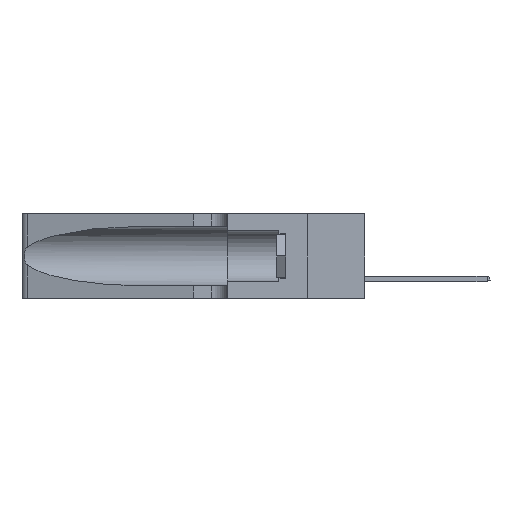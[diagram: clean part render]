
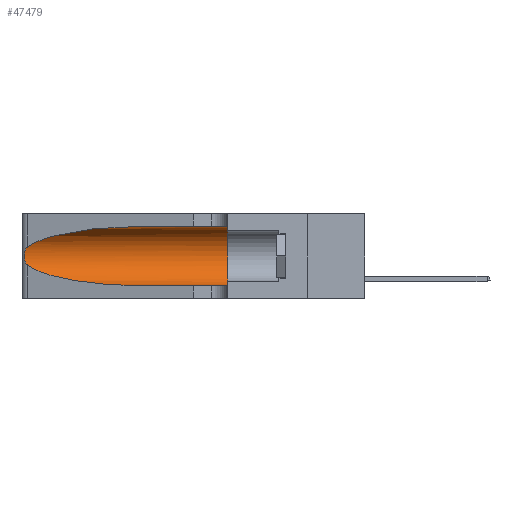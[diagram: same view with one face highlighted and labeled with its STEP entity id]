
A CAD part, left-side view. The second image highlights one B-rep face of the part: STEP entity #47479.
In plain terms, the highlighted cylindrical face has radius 3.308 mm (diameter 6.617 mm), a partial arc.
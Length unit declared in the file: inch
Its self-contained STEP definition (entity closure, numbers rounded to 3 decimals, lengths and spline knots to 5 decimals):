
#219 =( BOUNDED_CURVE ( )  B_SPLINE_CURVE ( 3, ( #15492, #26360, #33299, #37040 ),
 .UNSPECIFIED., .F., .T. ) 
 B_SPLINE_CURVE_WITH_KNOTS ( ( 4, 4 ),
 ( 1.5708, 2.84003 ),
 .UNSPECIFIED. ) 
 CURVE ( )  GEOMETRIC_REPRESENTATION_ITEM ( )  RATIONAL_B_SPLINE_CURVE ( ( 1., 0.87, 0.87, 1. ) ) 
 REPRESENTATION_ITEM ( '' )  );
#1433 = CARTESIAN_POINT ( 'NONE',  ( 0.2373, 1.15595, 0.08982 ) ) ;
#1579 = VERTEX_POINT ( 'NONE', #8436 ) ;
#2025 = DIRECTION ( 'NONE',  ( 0., 1., 0. ) ) ;
#2795 = ORIENTED_EDGE ( 'NONE', *, *, #7237, .F. ) ;
#5090 = LINE ( 'NONE', #26822, #35211 ) ;
#5856 = EDGE_CURVE ( 'NONE', #35575, #1579, #219, .T. ) ;
#6345 = CARTESIAN_POINT ( 'NONE',  ( 0.1305, 1.61858, 0.05475 ) ) ;
#6360 = FACE_OUTER_BOUND ( 'NONE', #33019, .T. ) ;
#6523 = ORIENTED_EDGE ( 'NONE', *, *, #47798, .F. ) ;
#6576 = CARTESIAN_POINT ( 'NONE',  ( 0.26017, 1.23833, 0.17102 ) ) ;
#6625 = DIRECTION ( 'NONE',  ( 0., -1., 0. ) ) ;
#6872 = CARTESIAN_POINT ( 'NONE',  ( 0.25555, 1.22993, 0.14849 ) ) ;
#7237 = EDGE_CURVE ( 'NONE', #11535, #20867, #25740, .T. ) ;
#8436 = CARTESIAN_POINT ( 'NONE',  ( 0.25487, 1.22718, 0.22369 ) ) ;
#9831 = EDGE_CURVE ( 'NONE', #43937, #15909, #36187, .T. ) ;
#10055 = AXIS2_PLACEMENT_3D ( 'NONE', #39849, #6625, #10306 ) ;
#10306 = DIRECTION ( 'NONE',  ( 0., 0., -1. ) ) ;
#10555 = CARTESIAN_POINT ( 'NONE',  ( 0.25789, 1.23486, 0.15765 ) ) ;
#11535 = VERTEX_POINT ( 'NONE', #21800 ) ;
#13190 = CARTESIAN_POINT ( 'NONE',  ( 0.25555, 1.22994, 0.2215 ) ) ;
#13523 = ORIENTED_EDGE ( 'NONE', *, *, #31975, .T. ) ;
#15492 = CARTESIAN_POINT ( 'NONE',  ( 0.1305, 0.72297, 0.31525 ) ) ;
#15909 = VERTEX_POINT ( 'NONE', #30723 ) ;
#16285 = CARTESIAN_POINT ( 'NONE',  ( 0.1305, 0.72297, 0.05475 ) ) ;
#16612 = CARTESIAN_POINT ( 'NONE',  ( 0.18966, 0.96281, 0.05475 ) ) ;
#16851 = DIRECTION ( 'NONE',  ( 0., 0., 1. ) ) ;
#18009 = CARTESIAN_POINT ( 'NONE',  ( 0.26018, 1.23835, 0.19895 ) ) ;
#18024 = ORIENTED_EDGE ( 'NONE', *, *, #45085, .T. ) ;
#19514 = CARTESIAN_POINT ( 'NONE',  ( 0.1305, 0.35, 0.05475 ) ) ;
#20793 = CYLINDRICAL_SURFACE ( 'NONE', #10055, 0.13025 ) ;
#20867 = VERTEX_POINT ( 'NONE', #19514 ) ;
#21800 = CARTESIAN_POINT ( 'NONE',  ( 0.1305, 0.35, 0.31525 ) ) ;
#22569 = ORIENTED_EDGE ( 'NONE', *, *, #5856, .T. ) ;
#24175 = CARTESIAN_POINT ( 'NONE',  ( 0.1305, 0.35, 0.185 ) ) ;
#24402 = CARTESIAN_POINT ( 'NONE',  ( 0.25854, 1.2359, 0.20912 ) ) ;
#25740 = CIRCLE ( 'NONE', #35718, 0.13025 ) ;
#25904 = CARTESIAN_POINT ( 'NONE',  ( 0.1305, 0.72297, 0.31525 ) ) ;
#26360 = CARTESIAN_POINT ( 'NONE',  ( 0.18966, 0.96281, 0.31525 ) ) ;
#26822 = CARTESIAN_POINT ( 'NONE',  ( 0.1305, 1.61858, 0.31525 ) ) ;
#27967 = CARTESIAN_POINT ( 'NONE',  ( 0.25487, 1.22718, 0.22369 ) ) ;
#28757 = CARTESIAN_POINT ( 'NONE',  ( 0.25487, 1.22718, 0.14631 ) ) ;
#28917 = CARTESIAN_POINT ( 'NONE',  ( 0.26075, 1.23896, 0.178 ) ) ;
#29241 = LINE ( 'NONE', #6345, #47222 ) ;
#30723 = CARTESIAN_POINT ( 'NONE',  ( 0.1305, 0.72297, 0.05475 ) ) ;
#31192 = CARTESIAN_POINT ( 'NONE',  ( 0.25487, 1.22718, 0.14631 ) ) ;
#31975 = EDGE_CURVE ( 'NONE', #15909, #20867, #29241, .T. ) ;
#32368 = B_SPLINE_CURVE_WITH_KNOTS ( 'NONE', 3,
 ( #27967, #13190, #43019, #46580, #24402, #18009, #47671, #28917, #6576, #40093, #10555, #47215, #6872, #28757 ),
 .UNSPECIFIED., .F., .F.,
 ( 4, 2, 2, 2, 2, 2, 4 ),
 ( 0., 0.00027, 0.00053, 0.00107, 0.0016, 0.00187, 0.00214 ),
 .UNSPECIFIED. ) ;
#32394 = DIRECTION ( 'NONE',  ( 0., -1., 0. ) ) ;
#33019 = EDGE_LOOP ( 'NONE', ( #22569, #18024, #46733, #13523, #2795, #6523 ) ) ;
#33299 = CARTESIAN_POINT ( 'NONE',  ( 0.2373, 1.15595, 0.28018 ) ) ;
#35211 = VECTOR ( 'NONE', #45572, 39.37008 ) ;
#35575 = VERTEX_POINT ( 'NONE', #25904 ) ;
#35718 = AXIS2_PLACEMENT_3D ( 'NONE', #24175, #2025, #16851 ) ;
#36187 =( BOUNDED_CURVE ( )  B_SPLINE_CURVE ( 3, ( #31192, #1433, #16612, #16285 ),
 .UNSPECIFIED., .F., .F. ) 
 B_SPLINE_CURVE_WITH_KNOTS ( ( 4, 4 ),
 ( 3.44316, 4.71239 ),
 .UNSPECIFIED. ) 
 CURVE ( )  GEOMETRIC_REPRESENTATION_ITEM ( )  RATIONAL_B_SPLINE_CURVE ( ( 1., 0.87, 0.87, 1. ) ) 
 REPRESENTATION_ITEM ( '' )  );
#36670 = CARTESIAN_POINT ( 'NONE',  ( 0.25487, 1.22718, 0.14631 ) ) ;
#37040 = CARTESIAN_POINT ( 'NONE',  ( 0.25487, 1.22718, 0.22369 ) ) ;
#39849 = CARTESIAN_POINT ( 'NONE',  ( 0.1305, 1.61858, 0.185 ) ) ;
#40093 = CARTESIAN_POINT ( 'NONE',  ( 0.25856, 1.23593, 0.16098 ) ) ;
#43019 = CARTESIAN_POINT ( 'NONE',  ( 0.25639, 1.23184, 0.21858 ) ) ;
#43937 = VERTEX_POINT ( 'NONE', #36670 ) ;
#45085 = EDGE_CURVE ( 'NONE', #1579, #43937, #32368, .T. ) ;
#45572 = DIRECTION ( 'NONE',  ( 0., -1., 0. ) ) ;
#46580 = CARTESIAN_POINT ( 'NONE',  ( 0.25787, 1.23484, 0.2124 ) ) ;
#46733 = ORIENTED_EDGE ( 'NONE', *, *, #9831, .T. ) ;
#47215 = CARTESIAN_POINT ( 'NONE',  ( 0.25639, 1.23186, 0.15144 ) ) ;
#47222 = VECTOR ( 'NONE', #32394, 39.37008 ) ;
#47479 = ADVANCED_FACE ( 'NONE', ( #6360 ), #20793, .F. ) ;
#47671 = CARTESIAN_POINT ( 'NONE',  ( 0.26075, 1.23896, 0.19203 ) ) ;
#47798 = EDGE_CURVE ( 'NONE', #35575, #11535, #5090, .T. ) ;
